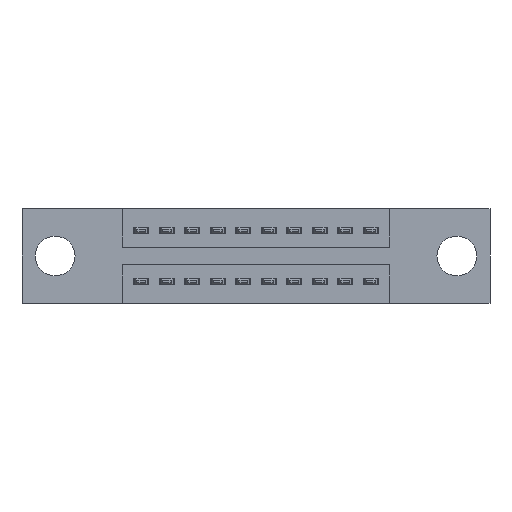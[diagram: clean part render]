
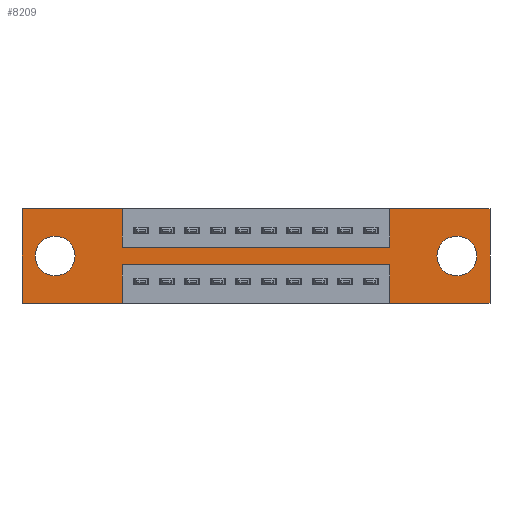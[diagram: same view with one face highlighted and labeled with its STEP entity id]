
A CAD part, front view. The second image highlights one B-rep face of the part: STEP entity #8209.
In plain terms, the highlighted planar face has unit normal (0, -1, 0).
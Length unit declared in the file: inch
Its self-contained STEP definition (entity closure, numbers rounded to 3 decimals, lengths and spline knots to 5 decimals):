
#1 = DIRECTION ( 'NONE',  ( 0., 0., 1. ) ) ;
#44 = VECTOR ( 'NONE', #6209, 39.37008 ) ;
#257 = PLANE ( 'NONE',  #3577 ) ;
#279 = ORIENTED_EDGE ( 'NONE', *, *, #5319, .F. ) ;
#540 = CIRCLE ( 'NONE', #2889, 0.078 ) ;
#636 = VECTOR ( 'NONE', #2882, 39.37008 ) ;
#924 = VECTOR ( 'NONE', #6846, 39.37008 ) ;
#1114 = DIRECTION ( 'NONE',  ( 0., -1., 0. ) ) ;
#1176 = VERTEX_POINT ( 'NONE', #10259 ) ;
#1197 = DIRECTION ( 'NONE',  ( 0., 0., 1. ) ) ;
#1222 = EDGE_CURVE ( 'NONE', #2592, #4216, #540, .T. ) ;
#1230 = DIRECTION ( 'NONE',  ( -1., 0., 0. ) ) ;
#1333 = VERTEX_POINT ( 'NONE', #6052 ) ;
#1397 = CARTESIAN_POINT ( 'NONE',  ( 0., 0., 0. ) ) ;
#1644 = CIRCLE ( 'NONE', #3895, 0.078 ) ;
#1654 = LINE ( 'NONE', #7817, #2668 ) ;
#1729 = DIRECTION ( 'NONE',  ( 1., 0., 0. ) ) ;
#1903 = CIRCLE ( 'NONE', #8065, 0.078 ) ;
#1972 = VERTEX_POINT ( 'NONE', #2992 ) ;
#1997 = CARTESIAN_POINT ( 'NONE',  ( 0., 0., -0.37 ) ) ;
#2239 = FACE_BOUND ( 'NONE', #4066, .T. ) ;
#2502 = DIRECTION ( 'NONE',  ( 0., 0., 1. ) ) ;
#2507 = VERTEX_POINT ( 'NONE', #4704 ) ;
#2525 = VECTOR ( 'NONE', #8830, 39.37008 ) ;
#2529 = FACE_OUTER_BOUND ( 'NONE', #7889, .T. ) ;
#2575 = VERTEX_POINT ( 'NONE', #3572 ) ;
#2591 = VERTEX_POINT ( 'NONE', #11051 ) ;
#2592 = VERTEX_POINT ( 'NONE', #3362 ) ;
#2615 = ORIENTED_EDGE ( 'NONE', *, *, #10685, .F. ) ;
#2654 = ORIENTED_EDGE ( 'NONE', *, *, #9675, .F. ) ;
#2668 = VECTOR ( 'NONE', #8753, 39.37008 ) ;
#2850 = EDGE_CURVE ( 'NONE', #2591, #1176, #9238, .T. ) ;
#2873 = VERTEX_POINT ( 'NONE', #3257 ) ;
#2882 = DIRECTION ( 'NONE',  ( -1., 0., 0. ) ) ;
#2889 = AXIS2_PLACEMENT_3D ( 'NONE', #5811, #8693, #6995 ) ;
#2992 = CARTESIAN_POINT ( 'NONE',  ( 1.4425, 0., -0.37 ) ) ;
#3040 = EDGE_CURVE ( 'NONE', #2873, #1972, #10955, .T. ) ;
#3123 = CARTESIAN_POINT ( 'NONE',  ( 0., 0., 0. ) ) ;
#3257 = CARTESIAN_POINT ( 'NONE',  ( 1.835, 0., -0.37 ) ) ;
#3277 = DIRECTION ( 'NONE',  ( 0., 0., 1. ) ) ;
#3362 = CARTESIAN_POINT ( 'NONE',  ( 1.705, 0., -0.107 ) ) ;
#3396 = EDGE_LOOP ( 'NONE', ( #5892, #6989 ) ) ;
#3400 = CARTESIAN_POINT ( 'NONE',  ( 1.4425, 0., -0.37 ) ) ;
#3443 = AXIS2_PLACEMENT_3D ( 'NONE', #6879, #6749, #1197 ) ;
#3493 = CARTESIAN_POINT ( 'NONE',  ( 0.3925, 0., 0. ) ) ;
#3523 = CARTESIAN_POINT ( 'NONE',  ( 0.3925, 0., -0.15 ) ) ;
#3547 = CARTESIAN_POINT ( 'NONE',  ( 0., 0., 0. ) ) ;
#3572 = CARTESIAN_POINT ( 'NONE',  ( 0.3925, 0., -0.15 ) ) ;
#3577 = AXIS2_PLACEMENT_3D ( 'NONE', #3965, #1114, #3927 ) ;
#3895 = AXIS2_PLACEMENT_3D ( 'NONE', #8984, #11790, #3277 ) ;
#3927 = DIRECTION ( 'NONE',  ( 0., 0., -1. ) ) ;
#3964 = DIRECTION ( 'NONE',  ( 0., 0., -1. ) ) ;
#3965 = CARTESIAN_POINT ( 'NONE',  ( 0., 0., -0.37 ) ) ;
#4066 = EDGE_LOOP ( 'NONE', ( #10354, #6537 ) ) ;
#4086 = ORIENTED_EDGE ( 'NONE', *, *, #3040, .F. ) ;
#4216 = VERTEX_POINT ( 'NONE', #10148 ) ;
#4242 = DIRECTION ( 'NONE',  ( 0., 1., 0. ) ) ;
#4303 = CARTESIAN_POINT ( 'NONE',  ( 1.4425, 0., -0.22 ) ) ;
#4494 = DIRECTION ( 'NONE',  ( -1., 0., 0. ) ) ;
#4604 = EDGE_CURVE ( 'NONE', #4216, #2592, #1903, .T. ) ;
#4633 = VECTOR ( 'NONE', #1230, 39.37008 ) ;
#4704 = CARTESIAN_POINT ( 'NONE',  ( 0.13, 0., -0.107 ) ) ;
#4801 = LINE ( 'NONE', #3123, #924 ) ;
#5001 = ORIENTED_EDGE ( 'NONE', *, *, #11319, .F. ) ;
#5002 = VECTOR ( 'NONE', #1729, 39.37008 ) ;
#5236 = LINE ( 'NONE', #1397, #6132 ) ;
#5270 = EDGE_CURVE ( 'NONE', #7286, #5453, #10925, .T. ) ;
#5319 = EDGE_CURVE ( 'NONE', #9125, #1333, #7454, .T. ) ;
#5453 = VERTEX_POINT ( 'NONE', #11171 ) ;
#5550 = ORIENTED_EDGE ( 'NONE', *, *, #8057, .F. ) ;
#5731 = VERTEX_POINT ( 'NONE', #9533 ) ;
#5798 = ORIENTED_EDGE ( 'NONE', *, *, #8492, .F. ) ;
#5811 = CARTESIAN_POINT ( 'NONE',  ( 1.705, 0., -0.185 ) ) ;
#5855 = CARTESIAN_POINT ( 'NONE',  ( 0.3925, 0., -0.22 ) ) ;
#5891 = VECTOR ( 'NONE', #2502, 39.37008 ) ;
#5892 = ORIENTED_EDGE ( 'NONE', *, *, #1222, .T. ) ;
#6004 = VECTOR ( 'NONE', #4494, 39.37008 ) ;
#6052 = CARTESIAN_POINT ( 'NONE',  ( 0., 0., 0. ) ) ;
#6132 = VECTOR ( 'NONE', #6923, 39.37008 ) ;
#6209 = DIRECTION ( 'NONE',  ( 0., 0., 1. ) ) ;
#6231 = CARTESIAN_POINT ( 'NONE',  ( 0.13, 0., -0.263 ) ) ;
#6268 = VERTEX_POINT ( 'NONE', #8864 ) ;
#6283 = LINE ( 'NONE', #11274, #6004 ) ;
#6537 = ORIENTED_EDGE ( 'NONE', *, *, #9815, .T. ) ;
#6749 = DIRECTION ( 'NONE',  ( 0., 1., 0. ) ) ;
#6838 = CARTESIAN_POINT ( 'NONE',  ( 1.835, 0., 0. ) ) ;
#6846 = DIRECTION ( 'NONE',  ( 1., 0., 0. ) ) ;
#6879 = CARTESIAN_POINT ( 'NONE',  ( 0.13, 0., -0.185 ) ) ;
#6909 = LINE ( 'NONE', #3400, #5891 ) ;
#6923 = DIRECTION ( 'NONE',  ( 1., 0., 0. ) ) ;
#6989 = ORIENTED_EDGE ( 'NONE', *, *, #4604, .T. ) ;
#6995 = DIRECTION ( 'NONE',  ( 0., 0., -1. ) ) ;
#7286 = VERTEX_POINT ( 'NONE', #4303 ) ;
#7453 = CARTESIAN_POINT ( 'NONE',  ( 0., 0., -0.37 ) ) ;
#7454 = LINE ( 'NONE', #3547, #44 ) ;
#7593 = CARTESIAN_POINT ( 'NONE',  ( 1.4425, 0., 0. ) ) ;
#7661 = VECTOR ( 'NONE', #10660, 39.37008 ) ;
#7668 = ORIENTED_EDGE ( 'NONE', *, *, #11063, .F. ) ;
#7676 = LINE ( 'NONE', #3523, #5002 ) ;
#7714 = EDGE_CURVE ( 'NONE', #2575, #2591, #7676, .T. ) ;
#7795 = CIRCLE ( 'NONE', #3443, 0.078 ) ;
#7817 = CARTESIAN_POINT ( 'NONE',  ( 0.3925, 0., -0.37 ) ) ;
#7889 = EDGE_LOOP ( 'NONE', ( #10894, #11525, #5798, #4086, #2654, #2615, #10640, #9682, #5550, #5001, #279, #7668 ) ) ;
#8057 = EDGE_CURVE ( 'NONE', #10994, #2575, #8554, .T. ) ;
#8065 = AXIS2_PLACEMENT_3D ( 'NONE', #9825, #4242, #3964 ) ;
#8124 = FACE_BOUND ( 'NONE', #3396, .T. ) ;
#8209 = ADVANCED_FACE ( 'NONE', ( #8124, #2239, #2529 ), #257, .T. ) ;
#8255 = LINE ( 'NONE', #6838, #2525 ) ;
#8492 = EDGE_CURVE ( 'NONE', #1972, #7286, #6909, .T. ) ;
#8554 = LINE ( 'NONE', #8814, #7661 ) ;
#8693 = DIRECTION ( 'NONE',  ( 0., 1., 0. ) ) ;
#8753 = DIRECTION ( 'NONE',  ( 0., 0., -1. ) ) ;
#8814 = CARTESIAN_POINT ( 'NONE',  ( 0.3925, 0., 0. ) ) ;
#8830 = DIRECTION ( 'NONE',  ( 0., 0., -1. ) ) ;
#8864 = CARTESIAN_POINT ( 'NONE',  ( 1.835, 0., 0. ) ) ;
#8984 = CARTESIAN_POINT ( 'NONE',  ( 0.13, 0., -0.185 ) ) ;
#9125 = VERTEX_POINT ( 'NONE', #1997 ) ;
#9190 = EDGE_CURVE ( 'NONE', #5453, #5731, #1654, .T. ) ;
#9238 = LINE ( 'NONE', #7593, #9378 ) ;
#9378 = VECTOR ( 'NONE', #1, 39.37008 ) ;
#9533 = CARTESIAN_POINT ( 'NONE',  ( 0.3925, 0., -0.37 ) ) ;
#9675 = EDGE_CURVE ( 'NONE', #6268, #2873, #8255, .T. ) ;
#9682 = ORIENTED_EDGE ( 'NONE', *, *, #7714, .F. ) ;
#9815 = EDGE_CURVE ( 'NONE', #10962, #2507, #1644, .T. ) ;
#9825 = CARTESIAN_POINT ( 'NONE',  ( 1.705, 0., -0.185 ) ) ;
#10129 = EDGE_CURVE ( 'NONE', #2507, #10962, #7795, .T. ) ;
#10148 = CARTESIAN_POINT ( 'NONE',  ( 1.705, 0., -0.263 ) ) ;
#10259 = CARTESIAN_POINT ( 'NONE',  ( 1.4425, 0., 0. ) ) ;
#10354 = ORIENTED_EDGE ( 'NONE', *, *, #10129, .T. ) ;
#10640 = ORIENTED_EDGE ( 'NONE', *, *, #2850, .F. ) ;
#10660 = DIRECTION ( 'NONE',  ( 0., 0., -1. ) ) ;
#10685 = EDGE_CURVE ( 'NONE', #1176, #6268, #4801, .T. ) ;
#10894 = ORIENTED_EDGE ( 'NONE', *, *, #9190, .F. ) ;
#10925 = LINE ( 'NONE', #5855, #4633 ) ;
#10955 = LINE ( 'NONE', #7453, #636 ) ;
#10962 = VERTEX_POINT ( 'NONE', #6231 ) ;
#10994 = VERTEX_POINT ( 'NONE', #3493 ) ;
#11051 = CARTESIAN_POINT ( 'NONE',  ( 1.4425, 0., -0.15 ) ) ;
#11063 = EDGE_CURVE ( 'NONE', #5731, #9125, #6283, .T. ) ;
#11171 = CARTESIAN_POINT ( 'NONE',  ( 0.3925, 0., -0.22 ) ) ;
#11274 = CARTESIAN_POINT ( 'NONE',  ( 0., 0., -0.37 ) ) ;
#11319 = EDGE_CURVE ( 'NONE', #1333, #10994, #5236, .T. ) ;
#11525 = ORIENTED_EDGE ( 'NONE', *, *, #5270, .F. ) ;
#11790 = DIRECTION ( 'NONE',  ( 0., 1., 0. ) ) ;
